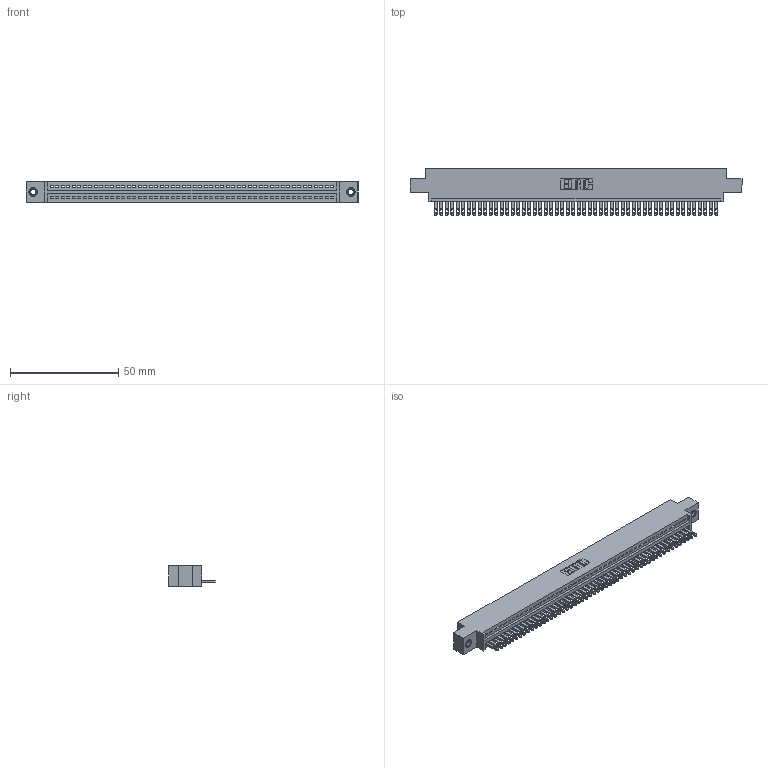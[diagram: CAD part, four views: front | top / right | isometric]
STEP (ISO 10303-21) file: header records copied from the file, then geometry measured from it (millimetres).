
FILE_DESCRIPTION (( 'STEP AP203' ), '1' );
FILE_NAME ('345-052-500-607.STEP', '2019-10-09T17:13:05', ( '' ), ( '' ), 'SwSTEP 2.0', 'SolidWorks 2016', '' );
FILE_SCHEMA (( 'CONFIG_CONTROL_DESIGN' ));
Length unit declared in the file: inch
Products named in the file (4): 345 Part_0.170 Offset - 0.156 Dia-TI; 345-250-001_345-250-005-103; 345-292-001_345-293-100; 345-052-500-607
Assembly tree (55 placements, depth 2):
  345-052-500-607
    345 Part_0.170 Offset - 0.156 Dia-TI
    345-292-001_345-293-100  x52
    345-250-001_345-250-005-103  x2
Bounding box: 153.29 x 21.51 x 9.4 mm (x, y, z)
Volume: 14546.7 mm3; surface area: 19743.1 mm2
Topology: 55 solids, 55 shells, 2998 faces, 9225 edges, 6142 vertices
Faces by surface type: plane 1884, cylinder 1098, cone 12, torus 4
Entity records: 39038 total; most frequent: CARTESIAN_POINT 6743, ORIENTED_EDGE 6722, DIRECTION 5903, EDGE_CURVE 3361, VECTOR 2997, LINE 2997, VERTEX_POINT 2236, AXIS2_PLACEMENT_3D 1453
